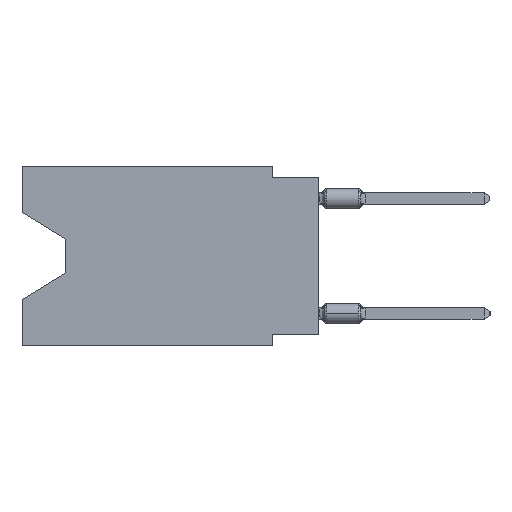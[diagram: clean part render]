
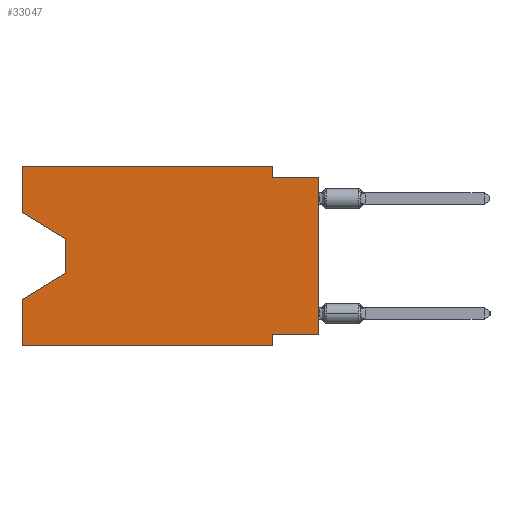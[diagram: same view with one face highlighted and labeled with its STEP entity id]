
A CAD part, left-side view. The second image highlights one B-rep face of the part: STEP entity #33047.
In plain terms, the highlighted planar face has unit normal (-1, 0, 0).
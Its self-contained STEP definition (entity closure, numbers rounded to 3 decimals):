
#228 = EDGE_CURVE ( 'NONE', #20137, #31118, #44210, .T. ) ;
#660 = CARTESIAN_POINT ( 'NONE',  ( 0., 16.383, -2.546 ) ) ;
#1078 = CARTESIAN_POINT ( 'NONE',  ( 0., 13.97, -5.893 ) ) ;
#1566 = VERTEX_POINT ( 'NONE', #35738 ) ;
#1598 = ORIENTED_EDGE ( 'NONE', *, *, #10188, .T. ) ;
#2434 = DIRECTION ( 'NONE',  ( 0., 1., 0. ) ) ;
#4269 = VECTOR ( 'NONE', #46483, 1000. ) ;
#4858 = CARTESIAN_POINT ( 'NONE',  ( 0., 16.383, -7.36 ) ) ;
#5434 = DIRECTION ( 'NONE',  ( 0., -1., 0. ) ) ;
#6673 = CARTESIAN_POINT ( 'NONE',  ( 0., 16.383, 0. ) ) ;
#7086 = CARTESIAN_POINT ( 'NONE',  ( 0., 2.54, 0. ) ) ;
#7349 = DIRECTION ( 'NONE',  ( 1., 0., 0. ) ) ;
#7398 = VERTEX_POINT ( 'NONE', #30424 ) ;
#7673 = VECTOR ( 'NONE', #26385, 1000. ) ;
#8413 = VECTOR ( 'NONE', #40352, 1000. ) ;
#9051 = VECTOR ( 'NONE', #40657, 1000. ) ;
#9158 = CARTESIAN_POINT ( 'NONE',  ( 0., 16.383, -9.906 ) ) ;
#9404 = CARTESIAN_POINT ( 'NONE',  ( 0., 16.383, 0. ) ) ;
#9744 = EDGE_CURVE ( 'NONE', #16702, #32385, #53718, .T. ) ;
#10188 = EDGE_CURVE ( 'NONE', #17611, #16702, #47442, .T. ) ;
#10963 = CARTESIAN_POINT ( 'NONE',  ( 0., 2.54, -9.906 ) ) ;
#11555 = VERTEX_POINT ( 'NONE', #39428 ) ;
#12849 = DIRECTION ( 'NONE',  ( 0., -1., 0. ) ) ;
#13100 = VERTEX_POINT ( 'NONE', #4858 ) ;
#13146 = CARTESIAN_POINT ( 'NONE',  ( 0., 13.97, -4.013 ) ) ;
#13401 = LINE ( 'NONE', #30393, #47806 ) ;
#13491 = ORIENTED_EDGE ( 'NONE', *, *, #50063, .T. ) ;
#13794 = CARTESIAN_POINT ( 'NONE',  ( 0., 2.54, -9.271 ) ) ;
#14230 = VECTOR ( 'NONE', #2434, 1000. ) ;
#14418 = EDGE_CURVE ( 'NONE', #31118, #34171, #46712, .T. ) ;
#14892 = VECTOR ( 'NONE', #36989, 1000. ) ;
#15354 = ORIENTED_EDGE ( 'NONE', *, *, #228, .F. ) ;
#16702 = VERTEX_POINT ( 'NONE', #13146 ) ;
#17257 = VECTOR ( 'NONE', #17981, 1000. ) ;
#17484 = LINE ( 'NONE', #9404, #7673 ) ;
#17611 = VERTEX_POINT ( 'NONE', #50571 ) ;
#17981 = DIRECTION ( 'NONE',  ( 0., 0., 1. ) ) ;
#19007 = EDGE_LOOP ( 'NONE', ( #1598, #49658, #39918, #36753, #13491, #44687, #15354, #33578, #54902, #31616, #50902, #30080 ) ) ;
#19580 = FACE_OUTER_BOUND ( 'NONE', #19007, .T. ) ;
#19729 = LINE ( 'NONE', #31722, #8413 ) ;
#19990 = EDGE_CURVE ( 'NONE', #17611, #1566, #27844, .T. ) ;
#20137 = VERTEX_POINT ( 'NONE', #39238 ) ;
#22132 = LINE ( 'NONE', #51928, #37154 ) ;
#23448 = EDGE_CURVE ( 'NONE', #24173, #13100, #41015, .T. ) ;
#24173 = VERTEX_POINT ( 'NONE', #9158 ) ;
#24530 = EDGE_CURVE ( 'NONE', #20137, #11555, #34980, .T. ) ;
#24994 = EDGE_CURVE ( 'NONE', #32385, #13100, #19729, .T. ) ;
#25422 = EDGE_CURVE ( 'NONE', #1566, #45129, #17484, .T. ) ;
#26385 = DIRECTION ( 'NONE',  ( 0., -1., 0. ) ) ;
#27844 = LINE ( 'NONE', #6673, #9051 ) ;
#28727 = CARTESIAN_POINT ( 'NONE',  ( 0., 2.54, 0. ) ) ;
#30080 = ORIENTED_EDGE ( 'NONE', *, *, #19990, .F. ) ;
#30393 = CARTESIAN_POINT ( 'NONE',  ( 0., 0., -0.635 ) ) ;
#30424 = CARTESIAN_POINT ( 'NONE',  ( 0., 2.54, -0.635 ) ) ;
#31118 = VERTEX_POINT ( 'NONE', #13794 ) ;
#31616 = ORIENTED_EDGE ( 'NONE', *, *, #51512, .F. ) ;
#31722 = CARTESIAN_POINT ( 'NONE',  ( 0., 13.97, -5.893 ) ) ;
#31816 = CARTESIAN_POINT ( 'NONE',  ( 0., 16.383, 0. ) ) ;
#32385 = VERTEX_POINT ( 'NONE', #1078 ) ;
#33047 = ADVANCED_FACE ( 'NONE', ( #19580 ), #54668, .F. ) ;
#33578 = ORIENTED_EDGE ( 'NONE', *, *, #24530, .T. ) ;
#34171 = VERTEX_POINT ( 'NONE', #10963 ) ;
#34980 = LINE ( 'NONE', #51143, #17257 ) ;
#35738 = CARTESIAN_POINT ( 'NONE',  ( 0., 16.383, 0. ) ) ;
#35998 = DIRECTION ( 'NONE',  ( 0., 0., 1. ) ) ;
#36129 = CARTESIAN_POINT ( 'NONE',  ( 0., 0., -9.271 ) ) ;
#36753 = ORIENTED_EDGE ( 'NONE', *, *, #23448, .F. ) ;
#36773 = VECTOR ( 'NONE', #35998, 1000. ) ;
#36989 = DIRECTION ( 'NONE',  ( 0., 0., -1. ) ) ;
#37154 = VECTOR ( 'NONE', #5434, 1000. ) ;
#37730 = DIRECTION ( 'NONE',  ( 0., 0., -1. ) ) ;
#39238 = CARTESIAN_POINT ( 'NONE',  ( 0., 0., -9.271 ) ) ;
#39428 = CARTESIAN_POINT ( 'NONE',  ( 0., 0., -0.635 ) ) ;
#39918 = ORIENTED_EDGE ( 'NONE', *, *, #24994, .T. ) ;
#40352 = DIRECTION ( 'NONE',  ( 0., 0.855, -0.519 ) ) ;
#40657 = DIRECTION ( 'NONE',  ( 0., 0., 1. ) ) ;
#41015 = LINE ( 'NONE', #31816, #36773 ) ;
#41635 = LINE ( 'NONE', #7086, #46011 ) ;
#44210 = LINE ( 'NONE', #36129, #14230 ) ;
#44687 = ORIENTED_EDGE ( 'NONE', *, *, #14418, .F. ) ;
#45129 = VERTEX_POINT ( 'NONE', #28727 ) ;
#45210 = VECTOR ( 'NONE', #51335, 1000. ) ;
#46011 = VECTOR ( 'NONE', #37730, 1000. ) ;
#46483 = DIRECTION ( 'NONE',  ( 0., 0., -1. ) ) ;
#46712 = LINE ( 'NONE', #50599, #14892 ) ;
#47442 = LINE ( 'NONE', #660, #45210 ) ;
#47806 = VECTOR ( 'NONE', #12849, 1000. ) ;
#49658 = ORIENTED_EDGE ( 'NONE', *, *, #9744, .T. ) ;
#50063 = EDGE_CURVE ( 'NONE', #24173, #34171, #22132, .T. ) ;
#50571 = CARTESIAN_POINT ( 'NONE',  ( 0., 16.383, -2.546 ) ) ;
#50599 = CARTESIAN_POINT ( 'NONE',  ( 0., 2.54, -9.906 ) ) ;
#50902 = ORIENTED_EDGE ( 'NONE', *, *, #25422, .F. ) ;
#51143 = CARTESIAN_POINT ( 'NONE',  ( 0., 0., 0. ) ) ;
#51335 = DIRECTION ( 'NONE',  ( 0., -0.855, -0.519 ) ) ;
#51512 = EDGE_CURVE ( 'NONE', #45129, #7398, #41635, .T. ) ;
#51742 = CARTESIAN_POINT ( 'NONE',  ( 0., 13.97, -4.013 ) ) ;
#51928 = CARTESIAN_POINT ( 'NONE',  ( 0., 16.383, -9.906 ) ) ;
#51974 = AXIS2_PLACEMENT_3D ( 'NONE', #54402, #7349, #53838 ) ;
#52050 = EDGE_CURVE ( 'NONE', #7398, #11555, #13401, .T. ) ;
#53718 = LINE ( 'NONE', #51742, #4269 ) ;
#53838 = DIRECTION ( 'NONE',  ( 0., 0., -1. ) ) ;
#54402 = CARTESIAN_POINT ( 'NONE',  ( 0., 16.383, 0. ) ) ;
#54668 = PLANE ( 'NONE',  #51974 ) ;
#54902 = ORIENTED_EDGE ( 'NONE', *, *, #52050, .F. ) ;
